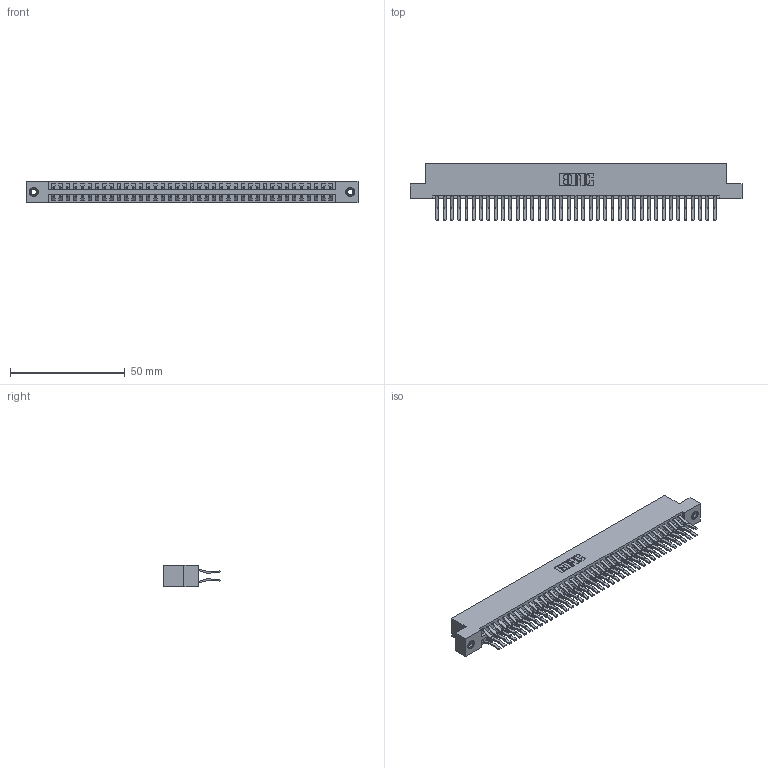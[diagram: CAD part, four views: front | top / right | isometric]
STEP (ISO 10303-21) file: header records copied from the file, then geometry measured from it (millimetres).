
FILE_DESCRIPTION (( 'STEP AP203' ), '1' );
FILE_NAME ('346-078-560-207.STEP', '2022-05-25T14:57:05', ( '' ), ( '' ), 'SwSTEP 2.0', 'SolidWorks 2020', '' );
FILE_SCHEMA (( 'CONFIG_CONTROL_DESIGN' ));
Length unit declared in the file: inch
Products named in the file (4): 346 Part_Flush Mounting Lugs - 0.156 Dia-TI; 346-078-560-207; 345-250-001_345-250-005-103; 345-292-001_560 Tail
Assembly tree (81 placements, depth 2):
  346-078-560-207
    346 Part_Flush Mounting Lugs - 0.156 Dia-TI
    345-292-001_560 Tail  x78
    345-250-001_345-250-005-103  x2
Bounding box: 144.4 x 24.78 x 9.4 mm (x, y, z)
Volume: 14555.1 mm3; surface area: 21357.6 mm2
Topology: 81 solids, 81 shells, 4394 faces, 13023 edges, 8570 vertices
Faces by surface type: plane 2838, cylinder 1540, cone 12, torus 4
Entity records: 27130 total; most frequent: CARTESIAN_POINT 4459, ORIENTED_EDGE 4386, DIRECTION 4011, EDGE_CURVE 2193, VECTOR 1881, LINE 1881, VERTEX_POINT 1456, AXIS2_PLACEMENT_3D 1065
